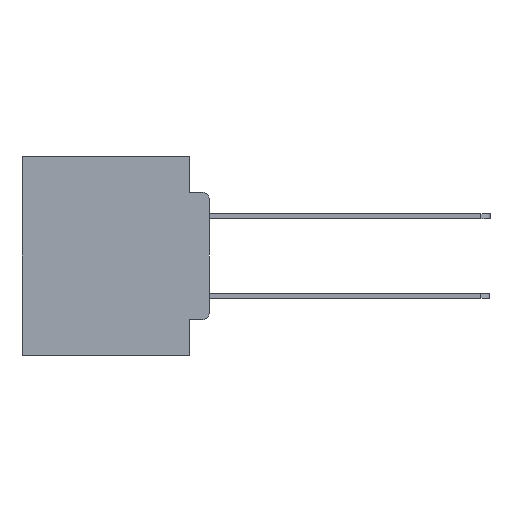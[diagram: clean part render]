
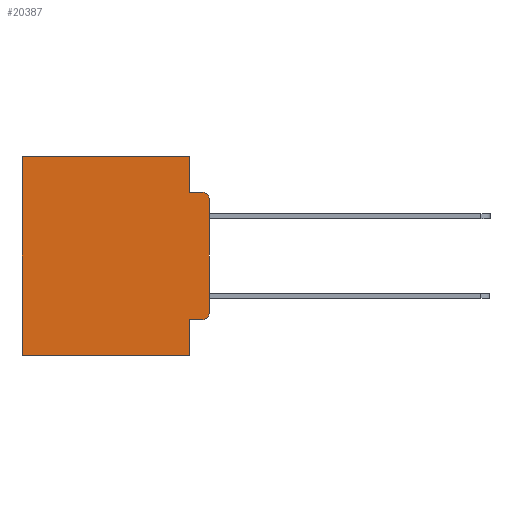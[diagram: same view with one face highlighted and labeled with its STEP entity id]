
A CAD part, left-side view. The second image highlights one B-rep face of the part: STEP entity #20387.
In plain terms, the highlighted planar face has unit normal (-1, 0, 0).
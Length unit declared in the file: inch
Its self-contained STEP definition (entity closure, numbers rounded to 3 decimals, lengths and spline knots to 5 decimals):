
#420 = VERTEX_POINT ( 'NONE', #17335 ) ;
#429 = VERTEX_POINT ( 'NONE', #27181 ) ;
#725 = EDGE_LOOP ( 'NONE', ( #4732, #25686, #1637, #6600, #18918, #4197, #22112, #2328, #29065, #17235 ) ) ;
#1257 = LINE ( 'NONE', #7669, #25344 ) ;
#1450 = EDGE_CURVE ( 'NONE', #6338, #15583, #9205, .T. ) ;
#1637 = ORIENTED_EDGE ( 'NONE', *, *, #27742, .F. ) ;
#2328 = ORIENTED_EDGE ( 'NONE', *, *, #2701, .F. ) ;
#2701 = EDGE_CURVE ( 'NONE', #17062, #6338, #1257, .T. ) ;
#3643 = CARTESIAN_POINT ( 'NONE',  ( 0.298, 0.051, -0.0885 ) ) ;
#4056 = CARTESIAN_POINT ( 'NONE',  ( 0.298, 0., -0.5 ) ) ;
#4197 = ORIENTED_EDGE ( 'NONE', *, *, #26625, .T. ) ;
#4286 = LINE ( 'NONE', #29167, #5078 ) ;
#4349 = EDGE_CURVE ( 'NONE', #17062, #429, #25586, .T. ) ;
#4732 = ORIENTED_EDGE ( 'NONE', *, *, #6188, .F. ) ;
#4775 = CARTESIAN_POINT ( 'NONE',  ( 0.298, 0.02, -0.0885 ) ) ;
#5078 = VECTOR ( 'NONE', #15542, 39.37008 ) ;
#5663 = VERTEX_POINT ( 'NONE', #25388 ) ;
#6066 = DIRECTION ( 'NONE',  ( 0., 0., -1. ) ) ;
#6188 = EDGE_CURVE ( 'NONE', #22285, #420, #16944, .T. ) ;
#6300 = CARTESIAN_POINT ( 'NONE',  ( 0.298, 0.02, -0.3915 ) ) ;
#6338 = VERTEX_POINT ( 'NONE', #18500 ) ;
#6600 = ORIENTED_EDGE ( 'NONE', *, *, #29269, .F. ) ;
#6626 = DIRECTION ( 'NONE',  ( 0., -1., 0. ) ) ;
#6734 = CARTESIAN_POINT ( 'NONE',  ( 0.298, 0.051, -0.4115 ) ) ;
#7669 = CARTESIAN_POINT ( 'NONE',  ( 0.298, 0.051, 0. ) ) ;
#7998 = DIRECTION ( 'NONE',  ( 0., 0., -1. ) ) ;
#8058 = LINE ( 'NONE', #13197, #24958 ) ;
#8469 = VECTOR ( 'NONE', #25925, 39.37008 ) ;
#8658 = DIRECTION ( 'NONE',  ( 0., 0., -1. ) ) ;
#8968 = DIRECTION ( 'NONE',  ( -1., 0., 0. ) ) ;
#9205 = LINE ( 'NONE', #4056, #8469 ) ;
#9829 = CARTESIAN_POINT ( 'NONE',  ( 0.298, 0.051, -0.0885 ) ) ;
#10242 = PLANE ( 'NONE',  #26003 ) ;
#12341 = CARTESIAN_POINT ( 'NONE',  ( 0.298, 0., -0.1085 ) ) ;
#12592 = LINE ( 'NONE', #23429, #30119 ) ;
#13197 = CARTESIAN_POINT ( 'NONE',  ( 0.298, 0.473, 0. ) ) ;
#13407 = VECTOR ( 'NONE', #6626, 39.37008 ) ;
#13883 = VERTEX_POINT ( 'NONE', #4775 ) ;
#13988 = EDGE_CURVE ( 'NONE', #22285, #13883, #28169, .T. ) ;
#14402 = EDGE_CURVE ( 'NONE', #15629, #5663, #4286, .T. ) ;
#15542 = DIRECTION ( 'NONE',  ( 0., 1., 0. ) ) ;
#15583 = VERTEX_POINT ( 'NONE', #21756 ) ;
#15629 = VERTEX_POINT ( 'NONE', #19561 ) ;
#16944 = LINE ( 'NONE', #18270, #28324 ) ;
#17062 = VERTEX_POINT ( 'NONE', #6734 ) ;
#17224 = CARTESIAN_POINT ( 'NONE',  ( 0.298, 0., 0. ) ) ;
#17235 = ORIENTED_EDGE ( 'NONE', *, *, #29087, .T. ) ;
#17335 = CARTESIAN_POINT ( 'NONE',  ( 0.298, 0., -0.3915 ) ) ;
#17767 = VECTOR ( 'NONE', #24566, 39.37008 ) ;
#18270 = CARTESIAN_POINT ( 'NONE',  ( 0.298, 0., 0. ) ) ;
#18500 = CARTESIAN_POINT ( 'NONE',  ( 0.298, 0.051, -0.5 ) ) ;
#18918 = ORIENTED_EDGE ( 'NONE', *, *, #14402, .T. ) ;
#19561 = CARTESIAN_POINT ( 'NONE',  ( 0.298, 0.051, 0. ) ) ;
#20387 = ADVANCED_FACE ( 'NONE', ( #28877 ), #10242, .F. ) ;
#21128 = DIRECTION ( 'NONE',  ( 0., 0., -1. ) ) ;
#21756 = CARTESIAN_POINT ( 'NONE',  ( 0.298, 0.473, -0.5 ) ) ;
#21782 = DIRECTION ( 'NONE',  ( 1., 0., 0. ) ) ;
#22112 = ORIENTED_EDGE ( 'NONE', *, *, #1450, .F. ) ;
#22285 = VERTEX_POINT ( 'NONE', #12341 ) ;
#22425 = DIRECTION ( 'NONE',  ( -1., 0., 0. ) ) ;
#22733 = CARTESIAN_POINT ( 'NONE',  ( 0.298, 0.02, -0.1085 ) ) ;
#23429 = CARTESIAN_POINT ( 'NONE',  ( 0.298, 0.051, 0. ) ) ;
#23828 = LINE ( 'NONE', #3643, #17767 ) ;
#24058 = VERTEX_POINT ( 'NONE', #9829 ) ;
#24459 = CIRCLE ( 'NONE', #29531, 0.02 ) ;
#24505 = DIRECTION ( 'NONE',  ( 0., 0., -1. ) ) ;
#24566 = DIRECTION ( 'NONE',  ( 0., -1., 0. ) ) ;
#24958 = VECTOR ( 'NONE', #26900, 39.37008 ) ;
#25046 = DIRECTION ( 'NONE',  ( 0., 0., -1. ) ) ;
#25344 = VECTOR ( 'NONE', #6066, 39.37008 ) ;
#25388 = CARTESIAN_POINT ( 'NONE',  ( 0.298, 0.473, 0. ) ) ;
#25586 = LINE ( 'NONE', #27319, #13407 ) ;
#25686 = ORIENTED_EDGE ( 'NONE', *, *, #13988, .T. ) ;
#25925 = DIRECTION ( 'NONE',  ( 0., 1., 0. ) ) ;
#26003 = AXIS2_PLACEMENT_3D ( 'NONE', #17224, #21782, #7998 ) ;
#26625 = EDGE_CURVE ( 'NONE', #5663, #15583, #8058, .T. ) ;
#26816 = AXIS2_PLACEMENT_3D ( 'NONE', #22733, #8968, #25046 ) ;
#26900 = DIRECTION ( 'NONE',  ( 0., 0., -1. ) ) ;
#27181 = CARTESIAN_POINT ( 'NONE',  ( 0.298, 0.02, -0.4115 ) ) ;
#27319 = CARTESIAN_POINT ( 'NONE',  ( 0.298, 0.051, -0.4115 ) ) ;
#27742 = EDGE_CURVE ( 'NONE', #24058, #13883, #23828, .T. ) ;
#28169 = CIRCLE ( 'NONE', #26816, 0.02 ) ;
#28324 = VECTOR ( 'NONE', #24505, 39.37008 ) ;
#28877 = FACE_OUTER_BOUND ( 'NONE', #725, .T. ) ;
#29065 = ORIENTED_EDGE ( 'NONE', *, *, #4349, .T. ) ;
#29087 = EDGE_CURVE ( 'NONE', #429, #420, #24459, .T. ) ;
#29167 = CARTESIAN_POINT ( 'NONE',  ( 0.298, 0., 0. ) ) ;
#29269 = EDGE_CURVE ( 'NONE', #15629, #24058, #12592, .T. ) ;
#29531 = AXIS2_PLACEMENT_3D ( 'NONE', #6300, #22425, #8658 ) ;
#30119 = VECTOR ( 'NONE', #21128, 39.37008 ) ;
